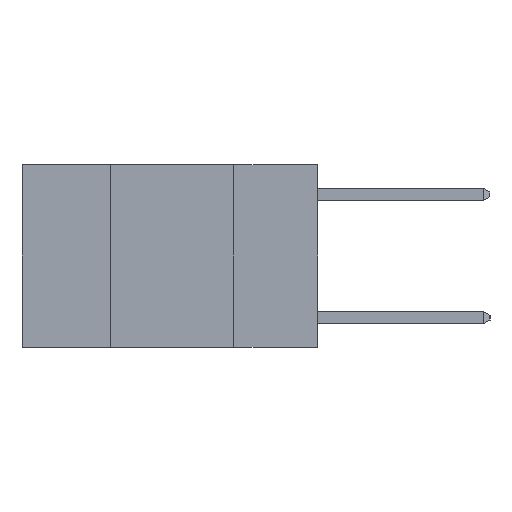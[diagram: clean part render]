
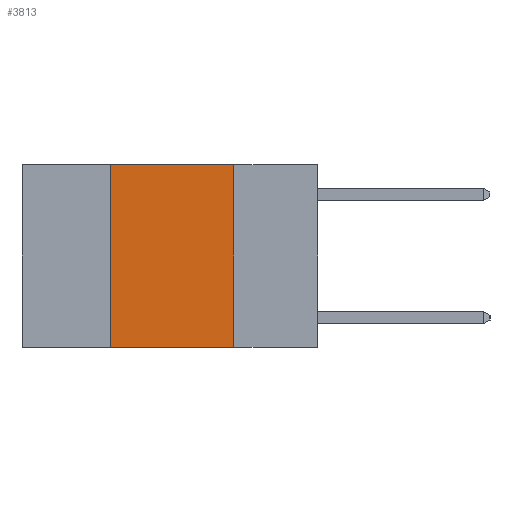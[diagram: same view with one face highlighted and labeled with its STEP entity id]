
A CAD part, left-side view. The second image highlights one B-rep face of the part: STEP entity #3813.
In plain terms, the highlighted planar face has unit normal (-1, 0, 0).
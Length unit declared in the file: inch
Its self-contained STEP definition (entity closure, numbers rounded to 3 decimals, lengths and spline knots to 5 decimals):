
#149 = DIRECTION ( 'NONE',  ( 0., 0., -1. ) ) ;
#178 = CARTESIAN_POINT ( 'NONE',  ( 0., 0.17, 0. ) ) ;
#204 = VECTOR ( 'NONE', #149, 39.37008 ) ;
#313 = ORIENTED_EDGE ( 'NONE', *, *, #6999, .F. ) ;
#389 = FACE_OUTER_BOUND ( 'NONE', #8666, .T. ) ;
#474 = DIRECTION ( 'NONE',  ( 0., 0., -1. ) ) ;
#506 = DIRECTION ( 'NONE',  ( 1., 0., 0. ) ) ;
#561 = CARTESIAN_POINT ( 'NONE',  ( 0., 0.6, 0. ) ) ;
#718 = PLANE ( 'NONE',  #3547 ) ;
#1321 = EDGE_CURVE ( 'NONE', #1977, #1416, #7987, .T. ) ;
#1416 = VERTEX_POINT ( 'NONE', #7515 ) ;
#1700 = LINE ( 'NONE', #4912, #8618 ) ;
#1977 = VERTEX_POINT ( 'NONE', #8453 ) ;
#2168 = ORIENTED_EDGE ( 'NONE', *, *, #3693, .T. ) ;
#2302 = LINE ( 'NONE', #178, #204 ) ;
#2686 = CARTESIAN_POINT ( 'NONE',  ( 0., 0.17, -0.37 ) ) ;
#3003 = VERTEX_POINT ( 'NONE', #2686 ) ;
#3247 = LINE ( 'NONE', #7531, #6564 ) ;
#3547 = AXIS2_PLACEMENT_3D ( 'NONE', #561, #506, #474 ) ;
#3693 = EDGE_CURVE ( 'NONE', #4855, #3003, #1700, .T. ) ;
#3813 = ADVANCED_FACE ( 'NONE', ( #389 ), #718, .F. ) ;
#3914 = ORIENTED_EDGE ( 'NONE', *, *, #4891, .F. ) ;
#3960 = VECTOR ( 'NONE', #8486, 39.37008 ) ;
#4770 = CARTESIAN_POINT ( 'NONE',  ( 0., 0.6, 0. ) ) ;
#4855 = VERTEX_POINT ( 'NONE', #7624 ) ;
#4891 = EDGE_CURVE ( 'NONE', #4855, #1977, #3247, .T. ) ;
#4912 = CARTESIAN_POINT ( 'NONE',  ( 0., 0.6, -0.37 ) ) ;
#4997 = DIRECTION ( 'NONE',  ( 0., -1., 0. ) ) ;
#5213 = ORIENTED_EDGE ( 'NONE', *, *, #1321, .F. ) ;
#6564 = VECTOR ( 'NONE', #7550, 39.37008 ) ;
#6999 = EDGE_CURVE ( 'NONE', #1416, #3003, #2302, .T. ) ;
#7515 = CARTESIAN_POINT ( 'NONE',  ( 0., 0.17, 0. ) ) ;
#7531 = CARTESIAN_POINT ( 'NONE',  ( 0., 0.42, 0. ) ) ;
#7550 = DIRECTION ( 'NONE',  ( 0., 0., 1. ) ) ;
#7624 = CARTESIAN_POINT ( 'NONE',  ( 0., 0.42, -0.37 ) ) ;
#7987 = LINE ( 'NONE', #4770, #3960 ) ;
#8453 = CARTESIAN_POINT ( 'NONE',  ( 0., 0.42, 0. ) ) ;
#8486 = DIRECTION ( 'NONE',  ( 0., -1., 0. ) ) ;
#8618 = VECTOR ( 'NONE', #4997, 39.37008 ) ;
#8666 = EDGE_LOOP ( 'NONE', ( #313, #5213, #3914, #2168 ) ) ;
